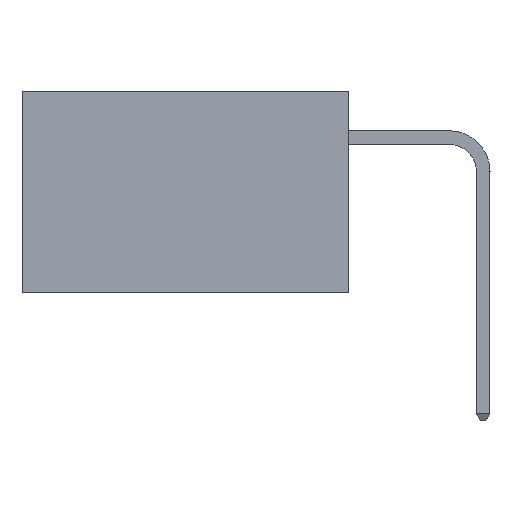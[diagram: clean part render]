
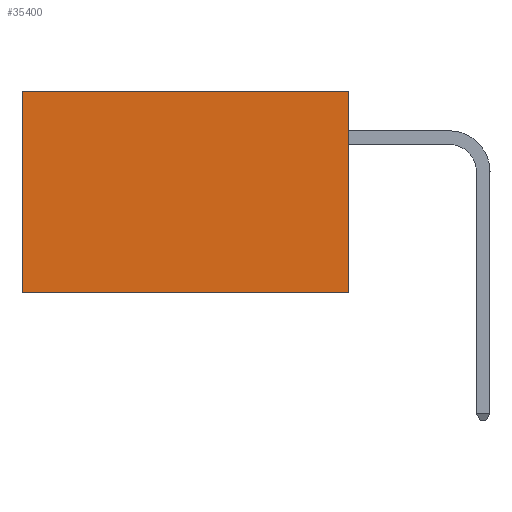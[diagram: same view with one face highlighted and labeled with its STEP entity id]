
A CAD part, left-side view. The second image highlights one B-rep face of the part: STEP entity #35400.
In plain terms, the highlighted planar face has unit normal (-1, 0, 0).
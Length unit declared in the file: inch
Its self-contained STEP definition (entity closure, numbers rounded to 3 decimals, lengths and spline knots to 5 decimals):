
#446 = LINE ( 'NONE', #25475, #28092 ) ;
#1472 = CARTESIAN_POINT ( 'NONE',  ( 0.2875, 0.6, 0. ) ) ;
#2293 = VERTEX_POINT ( 'NONE', #7737 ) ;
#5878 = ORIENTED_EDGE ( 'NONE', *, *, #31930, .F. ) ;
#6053 = CARTESIAN_POINT ( 'NONE',  ( 0.2875, 0., 0. ) ) ;
#7737 = CARTESIAN_POINT ( 'NONE',  ( 0.2875, 0.6, 0. ) ) ;
#7807 = VECTOR ( 'NONE', #26303, 39.37008 ) ;
#8296 = EDGE_CURVE ( 'NONE', #25271, #2293, #16649, .T. ) ;
#8854 = PLANE ( 'NONE',  #33612 ) ;
#11620 = DIRECTION ( 'NONE',  ( 0., 0., -1. ) ) ;
#12581 = CARTESIAN_POINT ( 'NONE',  ( 0.2875, 0., 0. ) ) ;
#13773 = EDGE_CURVE ( 'NONE', #25271, #17001, #446, .T. ) ;
#13937 = EDGE_CURVE ( 'NONE', #2293, #28725, #29834, .T. ) ;
#15364 = DIRECTION ( 'NONE',  ( 0., 1., 0. ) ) ;
#16585 = CARTESIAN_POINT ( 'NONE',  ( 0.2875, 0.6, -0.37 ) ) ;
#16649 = LINE ( 'NONE', #31886, #31341 ) ;
#17001 = VERTEX_POINT ( 'NONE', #27096 ) ;
#18629 = EDGE_LOOP ( 'NONE', ( #25784, #5878, #29061, #28108 ) ) ;
#20134 = CARTESIAN_POINT ( 'NONE',  ( 0.2875, 0., -0.37 ) ) ;
#20271 = VECTOR ( 'NONE', #22903, 39.37008 ) ;
#22903 = DIRECTION ( 'NONE',  ( 0., 1., 0. ) ) ;
#25271 = VERTEX_POINT ( 'NONE', #12581 ) ;
#25475 = CARTESIAN_POINT ( 'NONE',  ( 0.2875, 0., 0. ) ) ;
#25784 = ORIENTED_EDGE ( 'NONE', *, *, #13937, .T. ) ;
#26303 = DIRECTION ( 'NONE',  ( 0., 0., -1. ) ) ;
#27096 = CARTESIAN_POINT ( 'NONE',  ( 0.2875, 0., -0.37 ) ) ;
#28092 = VECTOR ( 'NONE', #33807, 39.37008 ) ;
#28108 = ORIENTED_EDGE ( 'NONE', *, *, #8296, .T. ) ;
#28725 = VERTEX_POINT ( 'NONE', #16585 ) ;
#29061 = ORIENTED_EDGE ( 'NONE', *, *, #13773, .F. ) ;
#29834 = LINE ( 'NONE', #1472, #7807 ) ;
#30794 = DIRECTION ( 'NONE',  ( 1., 0., 0. ) ) ;
#31341 = VECTOR ( 'NONE', #15364, 39.37008 ) ;
#31886 = CARTESIAN_POINT ( 'NONE',  ( 0.2875, 0., 0. ) ) ;
#31930 = EDGE_CURVE ( 'NONE', #17001, #28725, #34938, .T. ) ;
#32084 = FACE_OUTER_BOUND ( 'NONE', #18629, .T. ) ;
#33612 = AXIS2_PLACEMENT_3D ( 'NONE', #6053, #30794, #11620 ) ;
#33807 = DIRECTION ( 'NONE',  ( 0., 0., -1. ) ) ;
#34938 = LINE ( 'NONE', #20134, #20271 ) ;
#35400 = ADVANCED_FACE ( 'NONE', ( #32084 ), #8854, .F. ) ;
